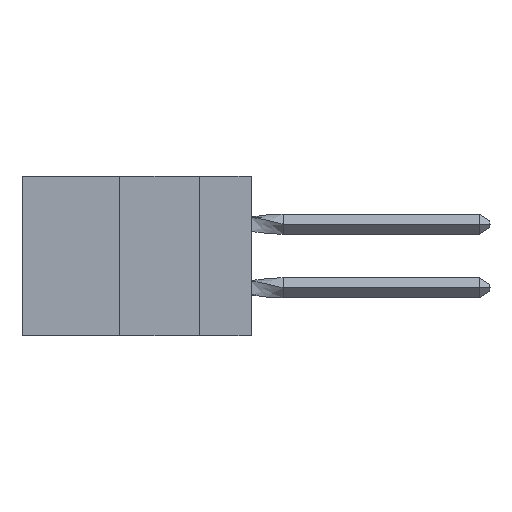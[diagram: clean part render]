
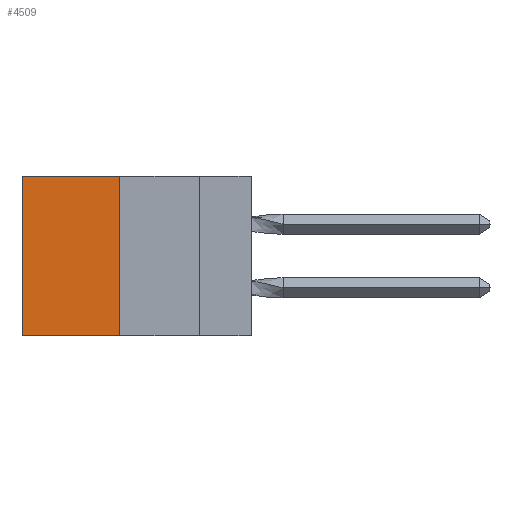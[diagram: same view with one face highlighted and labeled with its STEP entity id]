
A CAD part, left-side view. The second image highlights one B-rep face of the part: STEP entity #4509.
In plain terms, the highlighted planar face has unit normal (-1, 0, 0).
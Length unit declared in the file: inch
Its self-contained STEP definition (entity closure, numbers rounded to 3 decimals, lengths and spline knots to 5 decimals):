
#460 = CARTESIAN_POINT ( 'NONE',  ( 0.305, 0.413, -0.5 ) ) ;
#985 = VECTOR ( 'NONE', #2988, 39.37008 ) ;
#2203 = DIRECTION ( 'NONE',  ( 0., 0., -1. ) ) ;
#2851 = ORIENTED_EDGE ( 'NONE', *, *, #10170, .T. ) ;
#2988 = DIRECTION ( 'NONE',  ( 0., 0., -1. ) ) ;
#3662 = EDGE_LOOP ( 'NONE', ( #2851, #20181, #18226, #10228 ) ) ;
#3883 = CARTESIAN_POINT ( 'NONE',  ( 0.305, 0.413, 0. ) ) ;
#4371 = PLANE ( 'NONE',  #8770 ) ;
#4440 = DIRECTION ( 'NONE',  ( 0., 1., 0. ) ) ;
#4509 = ADVANCED_FACE ( 'NONE', ( #15059 ), #4371, .F. ) ;
#5588 = VECTOR ( 'NONE', #17511, 39.37008 ) ;
#5655 = VERTEX_POINT ( 'NONE', #11284 ) ;
#5721 = CARTESIAN_POINT ( 'NONE',  ( 0.305, 0.72, -0.5 ) ) ;
#8551 = CARTESIAN_POINT ( 'NONE',  ( 0.305, 0.72, -0.5 ) ) ;
#8770 = AXIS2_PLACEMENT_3D ( 'NONE', #21267, #13534, #2203 ) ;
#9129 = VECTOR ( 'NONE', #21250, 39.37008 ) ;
#9286 = CARTESIAN_POINT ( 'NONE',  ( 0.305, 0.413, -0.5 ) ) ;
#10170 = EDGE_CURVE ( 'NONE', #5655, #20421, #24040, .T. ) ;
#10228 = ORIENTED_EDGE ( 'NONE', *, *, #20146, .T. ) ;
#10267 = VERTEX_POINT ( 'NONE', #9286 ) ;
#11284 = CARTESIAN_POINT ( 'NONE',  ( 0.305, 0.72, 0. ) ) ;
#12585 = VECTOR ( 'NONE', #4440, 39.37008 ) ;
#13137 = EDGE_CURVE ( 'NONE', #10267, #20421, #20338, .T. ) ;
#13534 = DIRECTION ( 'NONE',  ( 1., 0., 0. ) ) ;
#14720 = LINE ( 'NONE', #23071, #9129 ) ;
#15059 = FACE_OUTER_BOUND ( 'NONE', #3662, .T. ) ;
#16406 = LINE ( 'NONE', #23526, #12585 ) ;
#17511 = DIRECTION ( 'NONE',  ( 0., 1., 0. ) ) ;
#18226 = ORIENTED_EDGE ( 'NONE', *, *, #23954, .F. ) ;
#20146 = EDGE_CURVE ( 'NONE', #22073, #5655, #16406, .T. ) ;
#20181 = ORIENTED_EDGE ( 'NONE', *, *, #13137, .F. ) ;
#20338 = LINE ( 'NONE', #460, #5588 ) ;
#20421 = VERTEX_POINT ( 'NONE', #5721 ) ;
#21250 = DIRECTION ( 'NONE',  ( 0., 0., -1. ) ) ;
#21267 = CARTESIAN_POINT ( 'NONE',  ( 0.305, 0.413, -0.5 ) ) ;
#22073 = VERTEX_POINT ( 'NONE', #3883 ) ;
#23071 = CARTESIAN_POINT ( 'NONE',  ( 0.305, 0.413, -0.5 ) ) ;
#23526 = CARTESIAN_POINT ( 'NONE',  ( 0.305, 0.413, 0. ) ) ;
#23954 = EDGE_CURVE ( 'NONE', #22073, #10267, #14720, .T. ) ;
#24040 = LINE ( 'NONE', #8551, #985 ) ;
